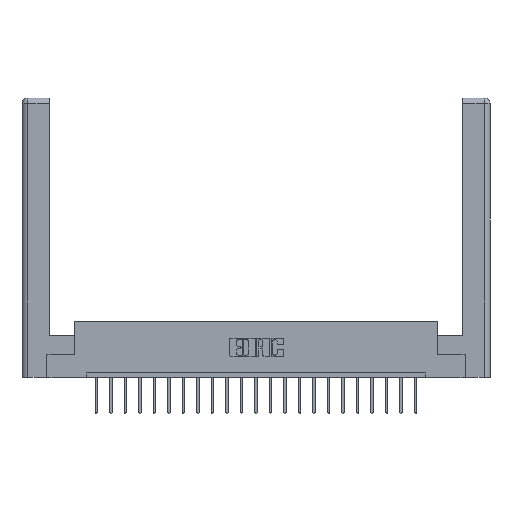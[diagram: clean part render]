
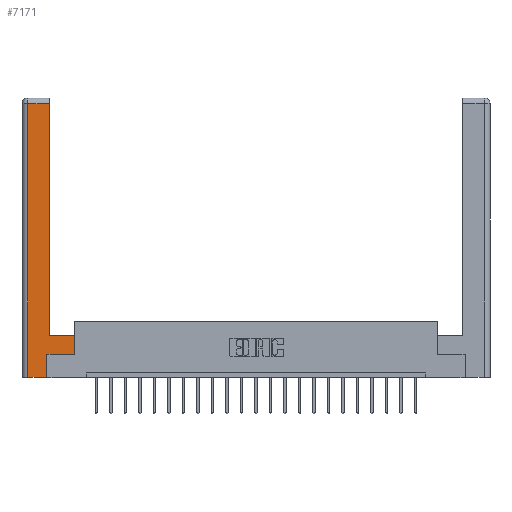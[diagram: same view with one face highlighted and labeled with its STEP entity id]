
A CAD part, top view. The second image highlights one B-rep face of the part: STEP entity #7171.
In plain terms, the highlighted planar face has unit normal (0, 0, 1).
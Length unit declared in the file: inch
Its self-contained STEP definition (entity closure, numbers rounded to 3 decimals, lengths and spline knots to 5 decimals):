
#314 = ORIENTED_EDGE ( 'NONE', *, *, #4807, .T. ) ;
#769 = CARTESIAN_POINT ( 'NONE',  ( 0.265, 0., 0. ) ) ;
#1001 = CARTESIAN_POINT ( 'NONE',  ( 0.565, 0.45, 0. ) ) ;
#1141 = CARTESIAN_POINT ( 'NONE',  ( 0.265, 0.245, 0. ) ) ;
#1323 = LINE ( 'NONE', #2266, #20639 ) ;
#1616 = CARTESIAN_POINT ( 'NONE',  ( 0.295, 2.94, 0. ) ) ;
#2266 = CARTESIAN_POINT ( 'NONE',  ( 0.0615, 2.94, 0. ) ) ;
#2275 = CARTESIAN_POINT ( 'NONE',  ( 0.565, 0.245, 0. ) ) ;
#2376 = VERTEX_POINT ( 'NONE', #5589 ) ;
#3019 = LINE ( 'NONE', #13735, #9937 ) ;
#3204 = LINE ( 'NONE', #20011, #5868 ) ;
#3666 = ORIENTED_EDGE ( 'NONE', *, *, #18676, .T. ) ;
#3859 = CARTESIAN_POINT ( 'NONE',  ( 0.565, 0.245, 0. ) ) ;
#3860 = EDGE_CURVE ( 'NONE', #2376, #7590, #3019, .T. ) ;
#3967 = DIRECTION ( 'NONE',  ( 1., 0., 0. ) ) ;
#4141 = DIRECTION ( 'NONE',  ( 1., 0., 0. ) ) ;
#4171 = DIRECTION ( 'NONE',  ( 0., 1., 0. ) ) ;
#4543 = VERTEX_POINT ( 'NONE', #17085 ) ;
#4793 = VECTOR ( 'NONE', #19819, 39.37008 ) ;
#4807 = EDGE_CURVE ( 'NONE', #5353, #4543, #11236, .T. ) ;
#5223 = CARTESIAN_POINT ( 'NONE',  ( 0.0615, 0., 0. ) ) ;
#5353 = VERTEX_POINT ( 'NONE', #7101 ) ;
#5381 = ORIENTED_EDGE ( 'NONE', *, *, #17752, .T. ) ;
#5589 = CARTESIAN_POINT ( 'NONE',  ( 0.565, 0.45, 0. ) ) ;
#5868 = VECTOR ( 'NONE', #18251, 39.37008 ) ;
#5910 = AXIS2_PLACEMENT_3D ( 'NONE', #14402, #8966, #19441 ) ;
#6198 = ORIENTED_EDGE ( 'NONE', *, *, #10516, .T. ) ;
#7101 = CARTESIAN_POINT ( 'NONE',  ( 0.265, 0., 0. ) ) ;
#7171 = ADVANCED_FACE ( 'NONE', ( #21549 ), #17721, .F. ) ;
#7272 = EDGE_CURVE ( 'NONE', #4543, #10430, #18368, .T. ) ;
#7590 = VERTEX_POINT ( 'NONE', #16543 ) ;
#8421 = DIRECTION ( 'NONE',  ( -1., 0., 0. ) ) ;
#8491 = LINE ( 'NONE', #1001, #17151 ) ;
#8903 = VECTOR ( 'NONE', #4141, 39.37008 ) ;
#8966 = DIRECTION ( 'NONE',  ( 0., 0., -1. ) ) ;
#9937 = VECTOR ( 'NONE', #8421, 39.37008 ) ;
#10430 = VERTEX_POINT ( 'NONE', #3859 ) ;
#10516 = EDGE_CURVE ( 'NONE', #10430, #2376, #8491, .T. ) ;
#11057 = CARTESIAN_POINT ( 'NONE',  ( 0.295, 3., 0. ) ) ;
#11236 = LINE ( 'NONE', #1141, #4793 ) ;
#11690 = ORIENTED_EDGE ( 'NONE', *, *, #13516, .T. ) ;
#13516 = EDGE_CURVE ( 'NONE', #22123, #20284, #3204, .T. ) ;
#13735 = CARTESIAN_POINT ( 'NONE',  ( 0.295, 0.45, 0. ) ) ;
#13937 = LINE ( 'NONE', #11057, #15558 ) ;
#14072 = VECTOR ( 'NONE', #3967, 39.37008 ) ;
#14402 = CARTESIAN_POINT ( 'NONE',  ( 0., 0., 0. ) ) ;
#14771 = DIRECTION ( 'NONE',  ( -1., 0., 0. ) ) ;
#14881 = CARTESIAN_POINT ( 'NONE',  ( 0.0615, 2.94, 0. ) ) ;
#15558 = VECTOR ( 'NONE', #4171, 39.37008 ) ;
#15599 = ORIENTED_EDGE ( 'NONE', *, *, #18448, .T. ) ;
#16528 = DIRECTION ( 'NONE',  ( 0., 1., 0. ) ) ;
#16543 = CARTESIAN_POINT ( 'NONE',  ( 0.295, 0.45, 0. ) ) ;
#17053 = ORIENTED_EDGE ( 'NONE', *, *, #7272, .T. ) ;
#17085 = CARTESIAN_POINT ( 'NONE',  ( 0.265, 0.245, 0. ) ) ;
#17151 = VECTOR ( 'NONE', #16528, 39.37008 ) ;
#17721 = PLANE ( 'NONE',  #5910 ) ;
#17752 = EDGE_CURVE ( 'NONE', #20284, #5353, #18646, .T. ) ;
#18142 = EDGE_LOOP ( 'NONE', ( #15599, #3666, #11690, #5381, #314, #17053, #6198, #22151 ) ) ;
#18251 = DIRECTION ( 'NONE',  ( 0., -1., 0. ) ) ;
#18368 = LINE ( 'NONE', #2275, #14072 ) ;
#18448 = EDGE_CURVE ( 'NONE', #7590, #20740, #13937, .T. ) ;
#18646 = LINE ( 'NONE', #769, #8903 ) ;
#18676 = EDGE_CURVE ( 'NONE', #20740, #22123, #1323, .T. ) ;
#19441 = DIRECTION ( 'NONE',  ( -1., 0., 0. ) ) ;
#19819 = DIRECTION ( 'NONE',  ( 0., 1., 0. ) ) ;
#20011 = CARTESIAN_POINT ( 'NONE',  ( 0.0615, 0., 0. ) ) ;
#20284 = VERTEX_POINT ( 'NONE', #5223 ) ;
#20639 = VECTOR ( 'NONE', #14771, 39.37008 ) ;
#20740 = VERTEX_POINT ( 'NONE', #1616 ) ;
#21549 = FACE_OUTER_BOUND ( 'NONE', #18142, .T. ) ;
#22123 = VERTEX_POINT ( 'NONE', #14881 ) ;
#22151 = ORIENTED_EDGE ( 'NONE', *, *, #3860, .T. ) ;
